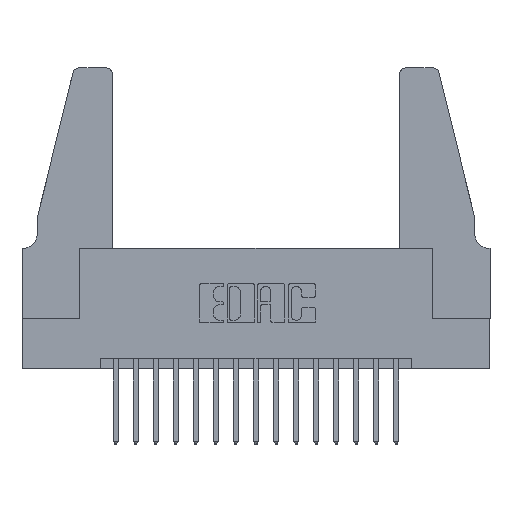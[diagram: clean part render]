
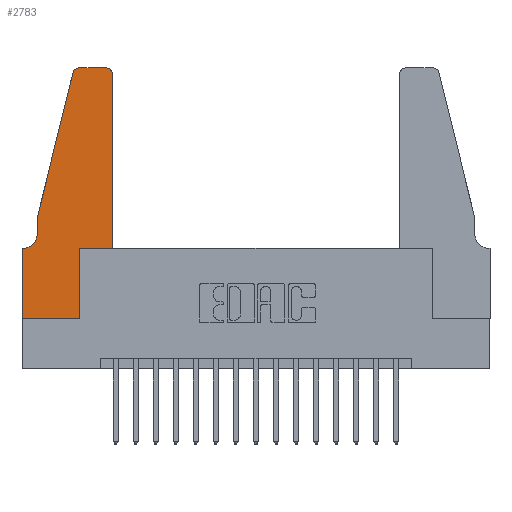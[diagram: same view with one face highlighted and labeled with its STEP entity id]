
A CAD part, top view. The second image highlights one B-rep face of the part: STEP entity #2783.
In plain terms, the highlighted planar face has unit normal (0, 0, 1).
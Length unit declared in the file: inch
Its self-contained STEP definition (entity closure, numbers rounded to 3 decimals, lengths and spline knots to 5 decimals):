
#288 = CARTESIAN_POINT ( 'NONE',  ( 0.4505, 0.35, 0.37 ) ) ;
#773 = DIRECTION ( 'NONE',  ( 0., 0., 1. ) ) ;
#938 = DIRECTION ( 'NONE',  ( -1., 0., 0. ) ) ;
#1101 = EDGE_CURVE ( 'NONE', #4129, #14528, #14277, .T. ) ;
#1269 = EDGE_CURVE ( 'NONE', #13395, #1378, #5000, .T. ) ;
#1351 = DIRECTION ( 'NONE',  ( 0., 1., 0. ) ) ;
#1378 = VERTEX_POINT ( 'NONE', #15876 ) ;
#1385 = EDGE_LOOP ( 'NONE', ( #2573, #13381, #6918, #3635, #7933, #7301, #3669, #3463, #15937, #6046, #7109, #9668 ) ) ;
#1412 = VERTEX_POINT ( 'NONE', #13784 ) ;
#1661 = VECTOR ( 'NONE', #4729, 39.37008 ) ;
#1737 = VECTOR ( 'NONE', #10640, 39.37008 ) ;
#1818 = EDGE_CURVE ( 'NONE', #8142, #10905, #10947, .T. ) ;
#1821 = DIRECTION ( 'NONE',  ( -1., 0., 0. ) ) ;
#2474 = CARTESIAN_POINT ( 'NONE',  ( 0.4205, 1.22, 0.37 ) ) ;
#2573 = ORIENTED_EDGE ( 'NONE', *, *, #1269, .T. ) ;
#2773 = VECTOR ( 'NONE', #13071, 39.37008 ) ;
#2783 = ADVANCED_FACE ( 'NONE', ( #17566 ), #7701, .T. ) ;
#2805 = EDGE_CURVE ( 'NONE', #1412, #7852, #3223, .T. ) ;
#2923 = CARTESIAN_POINT ( 'NONE',  ( 0.0055, 0.42, 0.37 ) ) ;
#3045 = DIRECTION ( 'NONE',  ( 0., 0., 1. ) ) ;
#3223 = LINE ( 'NONE', #9043, #2773 ) ;
#3336 = CARTESIAN_POINT ( 'NONE',  ( 0., 0., 0.37 ) ) ;
#3463 = ORIENTED_EDGE ( 'NONE', *, *, #16097, .T. ) ;
#3533 = AXIS2_PLACEMENT_3D ( 'NONE', #2923, #16615, #1821 ) ;
#3635 = ORIENTED_EDGE ( 'NONE', *, *, #16671, .T. ) ;
#3669 = ORIENTED_EDGE ( 'NONE', *, *, #2805, .T. ) ;
#3698 = AXIS2_PLACEMENT_3D ( 'NONE', #2474, #12014, #3897 ) ;
#3842 = CARTESIAN_POINT ( 'NONE',  ( 0.25487, 1.22718, 0.37 ) ) ;
#3897 = DIRECTION ( 'NONE',  ( 1., 0., 0. ) ) ;
#4129 = VERTEX_POINT ( 'NONE', #14371 ) ;
#4177 = LINE ( 'NONE', #288, #14955 ) ;
#4474 = DIRECTION ( 'NONE',  ( 0., -1., 0. ) ) ;
#4619 = EDGE_CURVE ( 'NONE', #14528, #7118, #4177, .T. ) ;
#4729 = DIRECTION ( 'NONE',  ( 1., 0., 0. ) ) ;
#4731 = VECTOR ( 'NONE', #10661, 39.37008 ) ;
#4736 = CARTESIAN_POINT ( 'NONE',  ( 0.2605, 1.25, 0.37 ) ) ;
#4940 = VERTEX_POINT ( 'NONE', #3842 ) ;
#4976 = EDGE_CURVE ( 'NONE', #10905, #1412, #16618, .T. ) ;
#5000 = LINE ( 'NONE', #4736, #11369 ) ;
#5236 = CARTESIAN_POINT ( 'NONE',  ( 0.0755, 0.5, 0.37 ) ) ;
#5715 = VERTEX_POINT ( 'NONE', #5236 ) ;
#6046 = ORIENTED_EDGE ( 'NONE', *, *, #4619, .T. ) ;
#6281 = EDGE_CURVE ( 'NONE', #9807, #13395, #16567, .T. ) ;
#6890 = CARTESIAN_POINT ( 'NONE',  ( 0.4505, 0.35, 0.37 ) ) ;
#6918 = ORIENTED_EDGE ( 'NONE', *, *, #11155, .T. ) ;
#7109 = ORIENTED_EDGE ( 'NONE', *, *, #9322, .T. ) ;
#7118 = VERTEX_POINT ( 'NONE', #17589 ) ;
#7301 = ORIENTED_EDGE ( 'NONE', *, *, #4976, .T. ) ;
#7701 = PLANE ( 'NONE',  #8043 ) ;
#7852 = VERTEX_POINT ( 'NONE', #13715 ) ;
#7933 = ORIENTED_EDGE ( 'NONE', *, *, #1818, .T. ) ;
#7962 = CIRCLE ( 'NONE', #14729, 0.03 ) ;
#8043 = AXIS2_PLACEMENT_3D ( 'NONE', #17056, #773, #10404 ) ;
#8142 = VERTEX_POINT ( 'NONE', #10394 ) ;
#8586 = DIRECTION ( 'NONE',  ( 1., 0., 0. ) ) ;
#9043 = CARTESIAN_POINT ( 'NONE',  ( 0., 0., 0.37 ) ) ;
#9127 = CARTESIAN_POINT ( 'NONE',  ( 0.2865, 0.35, 0.37 ) ) ;
#9309 = CARTESIAN_POINT ( 'NONE',  ( 0.0755, 0.5, 0.37 ) ) ;
#9322 = EDGE_CURVE ( 'NONE', #7118, #9807, #11763, .T. ) ;
#9342 = CARTESIAN_POINT ( 'NONE',  ( 0.0755, 0.35, 0.37 ) ) ;
#9668 = ORIENTED_EDGE ( 'NONE', *, *, #6281, .T. ) ;
#9807 = VERTEX_POINT ( 'NONE', #15906 ) ;
#10394 = CARTESIAN_POINT ( 'NONE',  ( 0.0755, 0.42, 0.37 ) ) ;
#10404 = DIRECTION ( 'NONE',  ( 1., 0., 0. ) ) ;
#10640 = DIRECTION ( 'NONE',  ( -1., 0., 0. ) ) ;
#10661 = DIRECTION ( 'NONE',  ( -0.239, -0.971, 0. ) ) ;
#10790 = CARTESIAN_POINT ( 'NONE',  ( 0.2865, 0.35, 0.37 ) ) ;
#10884 = VECTOR ( 'NONE', #4474, 39.37008 ) ;
#10905 = VERTEX_POINT ( 'NONE', #12817 ) ;
#10947 = CIRCLE ( 'NONE', #3533, 0.07 ) ;
#11155 = EDGE_CURVE ( 'NONE', #4940, #5715, #15496, .T. ) ;
#11211 = CARTESIAN_POINT ( 'NONE',  ( 0.284, 1.22, 0.37 ) ) ;
#11369 = VECTOR ( 'NONE', #938, 39.37008 ) ;
#11763 = LINE ( 'NONE', #6890, #15332 ) ;
#12014 = DIRECTION ( 'NONE',  ( 0., 0., 1. ) ) ;
#12535 = DIRECTION ( 'NONE',  ( 1., 0., 0. ) ) ;
#12559 = LINE ( 'NONE', #3336, #1661 ) ;
#12817 = CARTESIAN_POINT ( 'NONE',  ( 0.0055, 0.35, 0.37 ) ) ;
#12999 = DIRECTION ( 'NONE',  ( 0., 1., 0. ) ) ;
#13071 = DIRECTION ( 'NONE',  ( 0., -1., 0. ) ) ;
#13381 = ORIENTED_EDGE ( 'NONE', *, *, #15970, .T. ) ;
#13395 = VERTEX_POINT ( 'NONE', #14706 ) ;
#13715 = CARTESIAN_POINT ( 'NONE',  ( 0., 0., 0.37 ) ) ;
#13784 = CARTESIAN_POINT ( 'NONE',  ( 0., 0.35, 0.37 ) ) ;
#13909 = CARTESIAN_POINT ( 'NONE',  ( 0.0755, 0.5, 0.37 ) ) ;
#14277 = LINE ( 'NONE', #9127, #15146 ) ;
#14371 = CARTESIAN_POINT ( 'NONE',  ( 0.2865, 0., 0.37 ) ) ;
#14404 = LINE ( 'NONE', #13909, #10884 ) ;
#14528 = VERTEX_POINT ( 'NONE', #10790 ) ;
#14706 = CARTESIAN_POINT ( 'NONE',  ( 0.4205, 1.25, 0.37 ) ) ;
#14729 = AXIS2_PLACEMENT_3D ( 'NONE', #11211, #3045, #12535 ) ;
#14955 = VECTOR ( 'NONE', #8586, 39.37008 ) ;
#15146 = VECTOR ( 'NONE', #12999, 39.37008 ) ;
#15332 = VECTOR ( 'NONE', #1351, 39.37008 ) ;
#15496 = LINE ( 'NONE', #9309, #4731 ) ;
#15876 = CARTESIAN_POINT ( 'NONE',  ( 0.284, 1.25, 0.37 ) ) ;
#15906 = CARTESIAN_POINT ( 'NONE',  ( 0.4505, 1.22, 0.37 ) ) ;
#15937 = ORIENTED_EDGE ( 'NONE', *, *, #1101, .T. ) ;
#15970 = EDGE_CURVE ( 'NONE', #1378, #4940, #7962, .T. ) ;
#16097 = EDGE_CURVE ( 'NONE', #7852, #4129, #12559, .T. ) ;
#16567 = CIRCLE ( 'NONE', #3698, 0.03 ) ;
#16615 = DIRECTION ( 'NONE',  ( 0., 0., -1. ) ) ;
#16618 = LINE ( 'NONE', #9342, #1737 ) ;
#16671 = EDGE_CURVE ( 'NONE', #5715, #8142, #14404, .T. ) ;
#17056 = CARTESIAN_POINT ( 'NONE',  ( 0., 0.35, 0.37 ) ) ;
#17566 = FACE_OUTER_BOUND ( 'NONE', #1385, .T. ) ;
#17589 = CARTESIAN_POINT ( 'NONE',  ( 0.4505, 0.35, 0.37 ) ) ;
